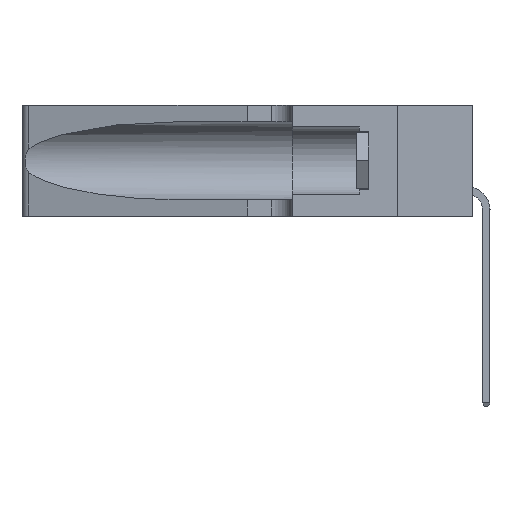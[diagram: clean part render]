
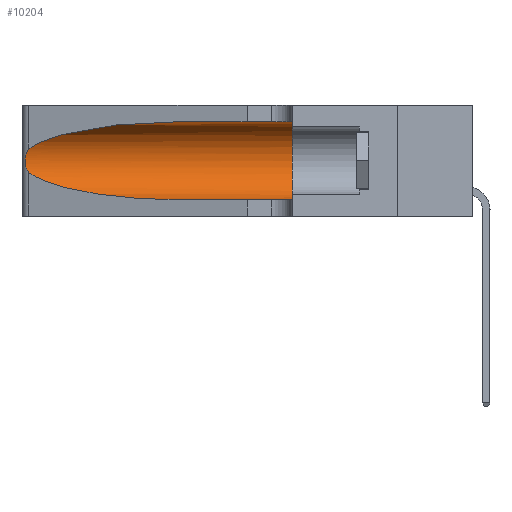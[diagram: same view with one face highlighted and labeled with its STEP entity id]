
A CAD part, left-side view. The second image highlights one B-rep face of the part: STEP entity #10204.
In plain terms, the highlighted cylindrical face has radius 3.308 mm (diameter 6.617 mm), a partial arc.
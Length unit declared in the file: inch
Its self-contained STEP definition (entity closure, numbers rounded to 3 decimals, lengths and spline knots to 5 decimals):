
#627 = DIRECTION ( 'NONE',  ( 0., 1., 0. ) ) ;
#631 = AXIS2_PLACEMENT_3D ( 'NONE', #6965, #18743, #11839 ) ;
#735 = CARTESIAN_POINT ( 'NONE',  ( 0.1305, 1.61858, 0.31525 ) ) ;
#1466 = CARTESIAN_POINT ( 'NONE',  ( 0.25787, 1.23484, 0.2124 ) ) ;
#1663 = CARTESIAN_POINT ( 'NONE',  ( 0.1305, 0.72297, 0.31525 ) ) ;
#2135 = ORIENTED_EDGE ( 'NONE', *, *, #10126, .T. ) ;
#2444 = CARTESIAN_POINT ( 'NONE',  ( 0.1305, 0.72297, 0.31525 ) ) ;
#3289 = CARTESIAN_POINT ( 'NONE',  ( 0.25789, 1.23486, 0.15765 ) ) ;
#3475 = CIRCLE ( 'NONE', #12900, 0.13025 ) ;
#3982 = CARTESIAN_POINT ( 'NONE',  ( 0.2373, 1.15595, 0.28018 ) ) ;
#4004 = CARTESIAN_POINT ( 'NONE',  ( 0.25487, 1.22718, 0.14631 ) ) ;
#4725 = VERTEX_POINT ( 'NONE', #10218 ) ;
#5148 = VERTEX_POINT ( 'NONE', #4004 ) ;
#5401 = EDGE_LOOP ( 'NONE', ( #17965, #11560, #2135, #12039, #10689, #9435 ) ) ;
#6747 = CARTESIAN_POINT ( 'NONE',  ( 0.1305, 1.61858, 0.05475 ) ) ;
#6965 = CARTESIAN_POINT ( 'NONE',  ( 0.1305, 1.61858, 0.185 ) ) ;
#7647 = B_SPLINE_CURVE_WITH_KNOTS ( 'NONE', 3,
 ( #12101, #11574, #10251, #1466, #13693, #16610, #18035, #12095, #9286, #10829, #3289, #12035, #15161, #16476 ),
 .UNSPECIFIED., .F., .F.,
 ( 4, 2, 2, 2, 2, 2, 4 ),
 ( 0., 0.00027, 0.00053, 0.00107, 0.0016, 0.00187, 0.00214 ),
 .UNSPECIFIED. ) ;
#7711 = DIRECTION ( 'NONE',  ( 0., 0., 1. ) ) ;
#8088 = DIRECTION ( 'NONE',  ( 0., -1., 0. ) ) ;
#8729 = DIRECTION ( 'NONE',  ( 0., -1., 0. ) ) ;
#8744 = CARTESIAN_POINT ( 'NONE',  ( 0.1305, 0.35, 0.05475 ) ) ;
#9286 = CARTESIAN_POINT ( 'NONE',  ( 0.26017, 1.23833, 0.17102 ) ) ;
#9435 = ORIENTED_EDGE ( 'NONE', *, *, #13043, .F. ) ;
#9885 = CARTESIAN_POINT ( 'NONE',  ( 0.2373, 1.15595, 0.08982 ) ) ;
#9912 = VECTOR ( 'NONE', #8729, 39.37008 ) ;
#10126 = EDGE_CURVE ( 'NONE', #5148, #4725, #10731, .T. ) ;
#10204 = ADVANCED_FACE ( 'NONE', ( #14538 ), #13599, .F. ) ;
#10218 = CARTESIAN_POINT ( 'NONE',  ( 0.1305, 0.72297, 0.05475 ) ) ;
#10251 = CARTESIAN_POINT ( 'NONE',  ( 0.25639, 1.23184, 0.21858 ) ) ;
#10279 = CARTESIAN_POINT ( 'NONE',  ( 0.25487, 1.22718, 0.14631 ) ) ;
#10689 = ORIENTED_EDGE ( 'NONE', *, *, #11918, .F. ) ;
#10731 =( BOUNDED_CURVE ( )  B_SPLINE_CURVE ( 3, ( #10279, #9885, #17658, #17135 ),
 .UNSPECIFIED., .F., .F. ) 
 B_SPLINE_CURVE_WITH_KNOTS ( ( 4, 4 ),
 ( 3.44316, 4.71239 ),
 .UNSPECIFIED. ) 
 CURVE ( )  GEOMETRIC_REPRESENTATION_ITEM ( )  RATIONAL_B_SPLINE_CURVE ( ( 1., 0.87, 0.87, 1. ) ) 
 REPRESENTATION_ITEM ( '' )  );
#10829 = CARTESIAN_POINT ( 'NONE',  ( 0.25856, 1.23593, 0.16098 ) ) ;
#11496 = EDGE_CURVE ( 'NONE', #18279, #5148, #7647, .T. ) ;
#11560 = ORIENTED_EDGE ( 'NONE', *, *, #11496, .T. ) ;
#11574 = CARTESIAN_POINT ( 'NONE',  ( 0.25555, 1.22994, 0.2215 ) ) ;
#11762 = VERTEX_POINT ( 'NONE', #8744 ) ;
#11839 = DIRECTION ( 'NONE',  ( 0., 0., -1. ) ) ;
#11906 = CARTESIAN_POINT ( 'NONE',  ( 0.1305, 0.35, 0.31525 ) ) ;
#11918 = EDGE_CURVE ( 'NONE', #13647, #11762, #3475, .T. ) ;
#12035 = CARTESIAN_POINT ( 'NONE',  ( 0.25639, 1.23186, 0.15144 ) ) ;
#12039 = ORIENTED_EDGE ( 'NONE', *, *, #18636, .T. ) ;
#12095 = CARTESIAN_POINT ( 'NONE',  ( 0.26075, 1.23896, 0.178 ) ) ;
#12101 = CARTESIAN_POINT ( 'NONE',  ( 0.25487, 1.22718, 0.22369 ) ) ;
#12650 = CARTESIAN_POINT ( 'NONE',  ( 0.25487, 1.22718, 0.22369 ) ) ;
#12678 = CARTESIAN_POINT ( 'NONE',  ( 0.18966, 0.96281, 0.31525 ) ) ;
#12900 = AXIS2_PLACEMENT_3D ( 'NONE', #16695, #627, #7711 ) ;
#13043 = EDGE_CURVE ( 'NONE', #18482, #13647, #17205, .T. ) ;
#13285 = VECTOR ( 'NONE', #8088, 39.37008 ) ;
#13529 =( BOUNDED_CURVE ( )  B_SPLINE_CURVE ( 3, ( #2444, #12678, #3982, #14220 ),
 .UNSPECIFIED., .F., .T. ) 
 B_SPLINE_CURVE_WITH_KNOTS ( ( 4, 4 ),
 ( 1.5708, 2.84003 ),
 .UNSPECIFIED. ) 
 CURVE ( )  GEOMETRIC_REPRESENTATION_ITEM ( )  RATIONAL_B_SPLINE_CURVE ( ( 1., 0.87, 0.87, 1. ) ) 
 REPRESENTATION_ITEM ( '' )  );
#13599 = CYLINDRICAL_SURFACE ( 'NONE', #631, 0.13025 ) ;
#13647 = VERTEX_POINT ( 'NONE', #11906 ) ;
#13693 = CARTESIAN_POINT ( 'NONE',  ( 0.25854, 1.2359, 0.20912 ) ) ;
#14220 = CARTESIAN_POINT ( 'NONE',  ( 0.25487, 1.22718, 0.22369 ) ) ;
#14245 = LINE ( 'NONE', #6747, #9912 ) ;
#14538 = FACE_OUTER_BOUND ( 'NONE', #5401, .T. ) ;
#15161 = CARTESIAN_POINT ( 'NONE',  ( 0.25555, 1.22993, 0.14849 ) ) ;
#16476 = CARTESIAN_POINT ( 'NONE',  ( 0.25487, 1.22718, 0.14631 ) ) ;
#16610 = CARTESIAN_POINT ( 'NONE',  ( 0.26018, 1.23835, 0.19895 ) ) ;
#16695 = CARTESIAN_POINT ( 'NONE',  ( 0.1305, 0.35, 0.185 ) ) ;
#16761 = EDGE_CURVE ( 'NONE', #18482, #18279, #13529, .T. ) ;
#17135 = CARTESIAN_POINT ( 'NONE',  ( 0.1305, 0.72297, 0.05475 ) ) ;
#17205 = LINE ( 'NONE', #735, #13285 ) ;
#17658 = CARTESIAN_POINT ( 'NONE',  ( 0.18966, 0.96281, 0.05475 ) ) ;
#17965 = ORIENTED_EDGE ( 'NONE', *, *, #16761, .T. ) ;
#18035 = CARTESIAN_POINT ( 'NONE',  ( 0.26075, 1.23896, 0.19203 ) ) ;
#18279 = VERTEX_POINT ( 'NONE', #12650 ) ;
#18482 = VERTEX_POINT ( 'NONE', #1663 ) ;
#18636 = EDGE_CURVE ( 'NONE', #4725, #11762, #14245, .T. ) ;
#18743 = DIRECTION ( 'NONE',  ( 0., -1., 0. ) ) ;
